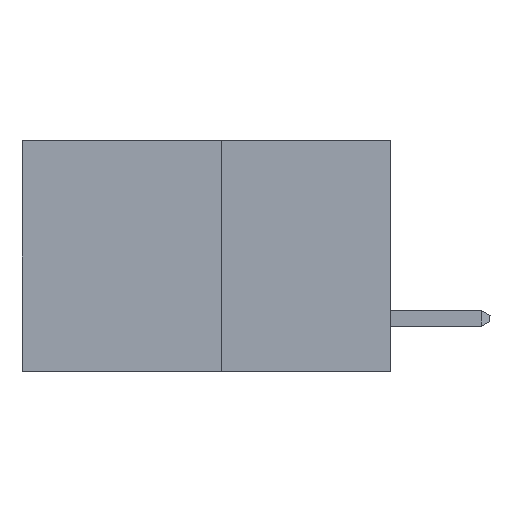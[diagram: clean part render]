
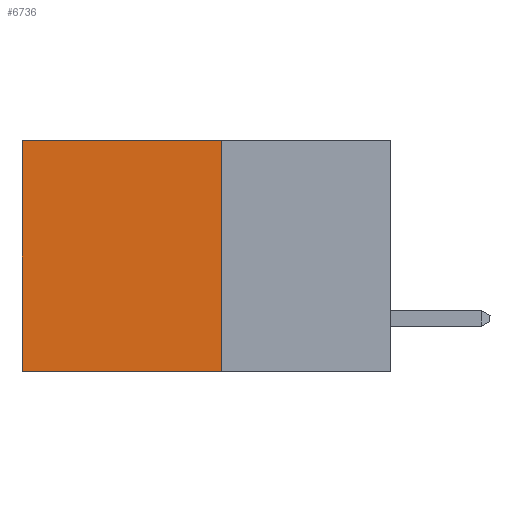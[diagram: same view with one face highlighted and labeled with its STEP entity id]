
A CAD part, left-side view. The second image highlights one B-rep face of the part: STEP entity #6736.
In plain terms, the highlighted planar face has unit normal (-1, 0, 0).
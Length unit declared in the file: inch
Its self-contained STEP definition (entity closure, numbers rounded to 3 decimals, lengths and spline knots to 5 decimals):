
#162 = CARTESIAN_POINT ( 'NONE',  ( 0.277, 0.59, -0.37 ) ) ;
#610 = LINE ( 'NONE', #3750, #6815 ) ;
#722 = DIRECTION ( 'NONE',  ( 0., 1., 0. ) ) ;
#1067 = CARTESIAN_POINT ( 'NONE',  ( 0.277, 0.27, -0.37 ) ) ;
#1326 = LINE ( 'NONE', #8129, #7506 ) ;
#1646 = EDGE_CURVE ( 'NONE', #8202, #6940, #1326, .T. ) ;
#1916 = DIRECTION ( 'NONE',  ( 0., 1., 0. ) ) ;
#1974 = EDGE_CURVE ( 'NONE', #8202, #8174, #6830, .T. ) ;
#1984 = ORIENTED_EDGE ( 'NONE', *, *, #7529, .F. ) ;
#1993 = VECTOR ( 'NONE', #722, 39.37008 ) ;
#2252 = AXIS2_PLACEMENT_3D ( 'NONE', #5897, #5857, #5847 ) ;
#2253 = ORIENTED_EDGE ( 'NONE', *, *, #1974, .T. ) ;
#2398 = VECTOR ( 'NONE', #1916, 39.37008 ) ;
#2520 = LINE ( 'NONE', #1067, #1993 ) ;
#3214 = CARTESIAN_POINT ( 'NONE',  ( 0.277, 0.27, -0.37 ) ) ;
#3607 = CARTESIAN_POINT ( 'NONE',  ( 0.277, 0.27, 0. ) ) ;
#3750 = CARTESIAN_POINT ( 'NONE',  ( 0.277, 0.59, -0.37 ) ) ;
#3912 = VERTEX_POINT ( 'NONE', #162 ) ;
#4189 = ORIENTED_EDGE ( 'NONE', *, *, #1646, .F. ) ;
#5157 = EDGE_CURVE ( 'NONE', #8174, #3912, #610, .T. ) ;
#5847 = DIRECTION ( 'NONE',  ( 0., 0., -1. ) ) ;
#5857 = DIRECTION ( 'NONE',  ( 1., 0., 0. ) ) ;
#5887 = PLANE ( 'NONE',  #2252 ) ;
#5897 = CARTESIAN_POINT ( 'NONE',  ( 0.277, 0.27, -0.37 ) ) ;
#6085 = EDGE_LOOP ( 'NONE', ( #10377, #1984, #4189, #2253 ) ) ;
#6641 = FACE_OUTER_BOUND ( 'NONE', #6085, .T. ) ;
#6736 = ADVANCED_FACE ( 'NONE', ( #6641 ), #5887, .F. ) ;
#6815 = VECTOR ( 'NONE', #8288, 39.37008 ) ;
#6830 = LINE ( 'NONE', #3607, #2398 ) ;
#6940 = VERTEX_POINT ( 'NONE', #3214 ) ;
#7305 = DIRECTION ( 'NONE',  ( 0., 0., -1. ) ) ;
#7506 = VECTOR ( 'NONE', #7305, 39.37008 ) ;
#7529 = EDGE_CURVE ( 'NONE', #6940, #3912, #2520, .T. ) ;
#7785 = CARTESIAN_POINT ( 'NONE',  ( 0.277, 0.59, 0. ) ) ;
#8129 = CARTESIAN_POINT ( 'NONE',  ( 0.277, 0.27, -0.37 ) ) ;
#8174 = VERTEX_POINT ( 'NONE', #7785 ) ;
#8202 = VERTEX_POINT ( 'NONE', #8700 ) ;
#8288 = DIRECTION ( 'NONE',  ( 0., 0., -1. ) ) ;
#8700 = CARTESIAN_POINT ( 'NONE',  ( 0.277, 0.27, 0. ) ) ;
#10377 = ORIENTED_EDGE ( 'NONE', *, *, #5157, .T. ) ;
